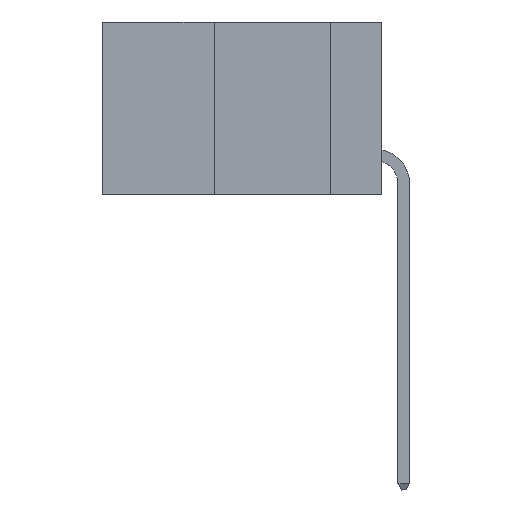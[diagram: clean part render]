
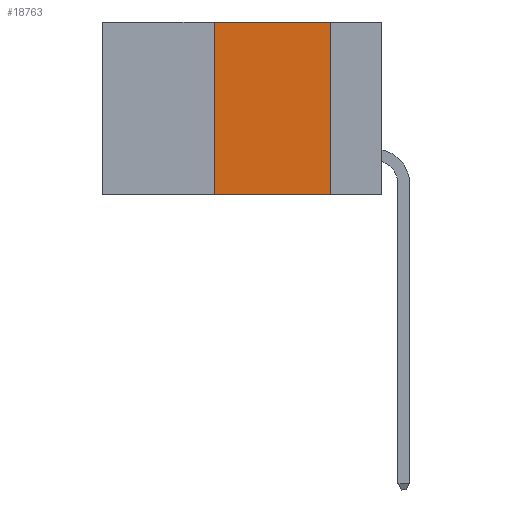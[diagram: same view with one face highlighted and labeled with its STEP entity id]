
A CAD part, left-side view. The second image highlights one B-rep face of the part: STEP entity #18763.
In plain terms, the highlighted planar face has unit normal (-1, 0, 0).
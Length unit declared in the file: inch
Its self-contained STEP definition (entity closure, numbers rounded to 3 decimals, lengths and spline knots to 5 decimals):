
#613 = VECTOR ( 'NONE', #6101, 39.37008 ) ;
#917 = CARTESIAN_POINT ( 'NONE',  ( 0., 0.36, -0.37 ) ) ;
#2877 = FACE_OUTER_BOUND ( 'NONE', #6547, .T. ) ;
#3160 = CARTESIAN_POINT ( 'NONE',  ( 0., 0.6, -0.37 ) ) ;
#3752 = CARTESIAN_POINT ( 'NONE',  ( 0., 0.36, 0. ) ) ;
#3878 = CARTESIAN_POINT ( 'NONE',  ( 0., 0.11, -0.37 ) ) ;
#3918 = LINE ( 'NONE', #15080, #15279 ) ;
#4597 = AXIS2_PLACEMENT_3D ( 'NONE', #18664, #15798, #6954 ) ;
#4704 = DIRECTION ( 'NONE',  ( 0., -1., 0. ) ) ;
#4729 = DIRECTION ( 'NONE',  ( 0., 0., -1. ) ) ;
#4866 = LINE ( 'NONE', #19270, #613 ) ;
#6101 = DIRECTION ( 'NONE',  ( 0., -1., 0. ) ) ;
#6127 = LINE ( 'NONE', #17912, #9093 ) ;
#6547 = EDGE_LOOP ( 'NONE', ( #10303, #10105, #10255, #10773 ) ) ;
#6954 = DIRECTION ( 'NONE',  ( 0., 0., -1. ) ) ;
#7584 = DIRECTION ( 'NONE',  ( 0., 0., 1. ) ) ;
#8320 = LINE ( 'NONE', #3160, #12282 ) ;
#9093 = VECTOR ( 'NONE', #7584, 39.37008 ) ;
#9559 = VERTEX_POINT ( 'NONE', #3752 ) ;
#9789 = VERTEX_POINT ( 'NONE', #3878 ) ;
#9924 = VERTEX_POINT ( 'NONE', #917 ) ;
#10105 = ORIENTED_EDGE ( 'NONE', *, *, #10847, .F. ) ;
#10255 = ORIENTED_EDGE ( 'NONE', *, *, #14901, .F. ) ;
#10303 = ORIENTED_EDGE ( 'NONE', *, *, #10905, .F. ) ;
#10502 = VERTEX_POINT ( 'NONE', #18547 ) ;
#10773 = ORIENTED_EDGE ( 'NONE', *, *, #17834, .T. ) ;
#10847 = EDGE_CURVE ( 'NONE', #9559, #10502, #4866, .T. ) ;
#10905 = EDGE_CURVE ( 'NONE', #10502, #9789, #3918, .T. ) ;
#12282 = VECTOR ( 'NONE', #4704, 39.37008 ) ;
#14901 = EDGE_CURVE ( 'NONE', #9924, #9559, #6127, .T. ) ;
#15080 = CARTESIAN_POINT ( 'NONE',  ( 0., 0.11, 0. ) ) ;
#15279 = VECTOR ( 'NONE', #4729, 39.37008 ) ;
#15737 = PLANE ( 'NONE',  #4597 ) ;
#15798 = DIRECTION ( 'NONE',  ( 1., 0., 0. ) ) ;
#17834 = EDGE_CURVE ( 'NONE', #9924, #9789, #8320, .T. ) ;
#17912 = CARTESIAN_POINT ( 'NONE',  ( 0., 0.36, 0. ) ) ;
#18547 = CARTESIAN_POINT ( 'NONE',  ( 0., 0.11, 0. ) ) ;
#18664 = CARTESIAN_POINT ( 'NONE',  ( 0., 0.6, 0. ) ) ;
#18763 = ADVANCED_FACE ( 'NONE', ( #2877 ), #15737, .F. ) ;
#19270 = CARTESIAN_POINT ( 'NONE',  ( 0., 0.6, 0. ) ) ;
